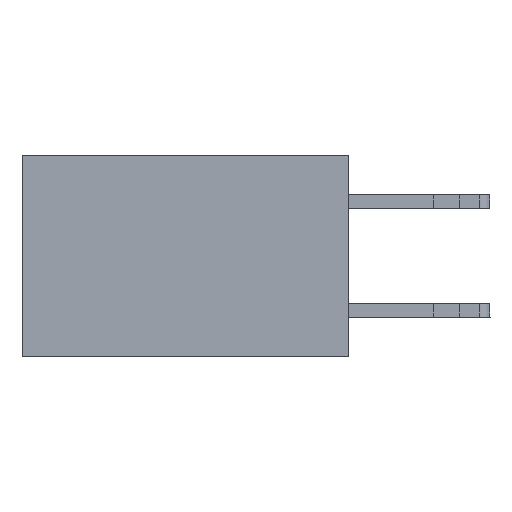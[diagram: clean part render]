
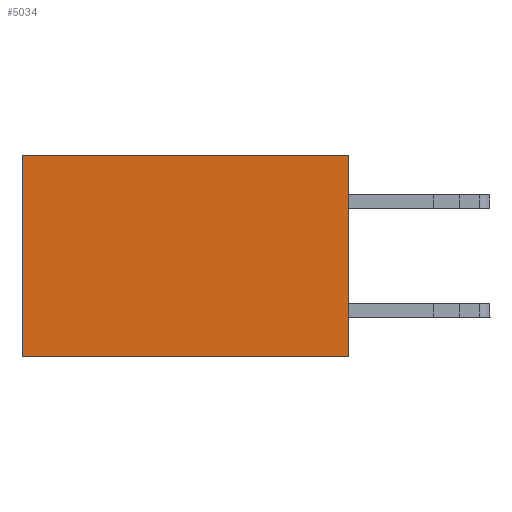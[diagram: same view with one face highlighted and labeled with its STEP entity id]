
A CAD part, left-side view. The second image highlights one B-rep face of the part: STEP entity #5034.
In plain terms, the highlighted planar face has unit normal (-1, 0, 0).
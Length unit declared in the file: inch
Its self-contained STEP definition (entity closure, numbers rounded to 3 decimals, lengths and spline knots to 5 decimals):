
#129 = DIRECTION ( 'NONE',  ( 0., 0., -1. ) ) ;
#212 = VERTEX_POINT ( 'NONE', #4460 ) ;
#299 = EDGE_LOOP ( 'NONE', ( #17224, #3297, #10816, #19948 ) ) ;
#642 = DIRECTION ( 'NONE',  ( 0., 0., -1. ) ) ;
#2184 = LINE ( 'NONE', #19967, #5011 ) ;
#2206 = DIRECTION ( 'NONE',  ( 1., 0., 0. ) ) ;
#3145 = VERTEX_POINT ( 'NONE', #5918 ) ;
#3297 = ORIENTED_EDGE ( 'NONE', *, *, #19921, .F. ) ;
#4211 = LINE ( 'NONE', #7822, #10308 ) ;
#4460 = CARTESIAN_POINT ( 'NONE',  ( 0.298, 0., 0. ) ) ;
#4643 = CARTESIAN_POINT ( 'NONE',  ( 0.298, 0., -0.37 ) ) ;
#5011 = VECTOR ( 'NONE', #14833, 39.37008 ) ;
#5034 = ADVANCED_FACE ( 'NONE', ( #21130 ), #13707, .F. ) ;
#5918 = CARTESIAN_POINT ( 'NONE',  ( 0.298, 0.6, 0. ) ) ;
#6234 = DIRECTION ( 'NONE',  ( 0., 1., 0. ) ) ;
#6985 = VECTOR ( 'NONE', #6234, 39.37008 ) ;
#7822 = CARTESIAN_POINT ( 'NONE',  ( 0.298, 0., 0. ) ) ;
#10308 = VECTOR ( 'NONE', #10971, 39.37008 ) ;
#10529 = VERTEX_POINT ( 'NONE', #20971 ) ;
#10816 = ORIENTED_EDGE ( 'NONE', *, *, #11296, .F. ) ;
#10971 = DIRECTION ( 'NONE',  ( 0., 1., 0. ) ) ;
#11296 = EDGE_CURVE ( 'NONE', #212, #19874, #14199, .T. ) ;
#11947 = EDGE_CURVE ( 'NONE', #212, #3145, #4211, .T. ) ;
#11996 = CARTESIAN_POINT ( 'NONE',  ( 0.298, 0., 0. ) ) ;
#13707 = PLANE ( 'NONE',  #16847 ) ;
#14199 = LINE ( 'NONE', #15281, #14454 ) ;
#14454 = VECTOR ( 'NONE', #642, 39.37008 ) ;
#14833 = DIRECTION ( 'NONE',  ( 0., 0., -1. ) ) ;
#15281 = CARTESIAN_POINT ( 'NONE',  ( 0.298, 0., 0. ) ) ;
#16028 = CARTESIAN_POINT ( 'NONE',  ( 0.298, 0., -0.37 ) ) ;
#16847 = AXIS2_PLACEMENT_3D ( 'NONE', #11996, #2206, #129 ) ;
#17224 = ORIENTED_EDGE ( 'NONE', *, *, #18555, .T. ) ;
#18042 = LINE ( 'NONE', #4643, #6985 ) ;
#18555 = EDGE_CURVE ( 'NONE', #3145, #10529, #2184, .T. ) ;
#19874 = VERTEX_POINT ( 'NONE', #16028 ) ;
#19921 = EDGE_CURVE ( 'NONE', #19874, #10529, #18042, .T. ) ;
#19948 = ORIENTED_EDGE ( 'NONE', *, *, #11947, .T. ) ;
#19967 = CARTESIAN_POINT ( 'NONE',  ( 0.298, 0.6, 0. ) ) ;
#20971 = CARTESIAN_POINT ( 'NONE',  ( 0.298, 0.6, -0.37 ) ) ;
#21130 = FACE_OUTER_BOUND ( 'NONE', #299, .T. ) ;
